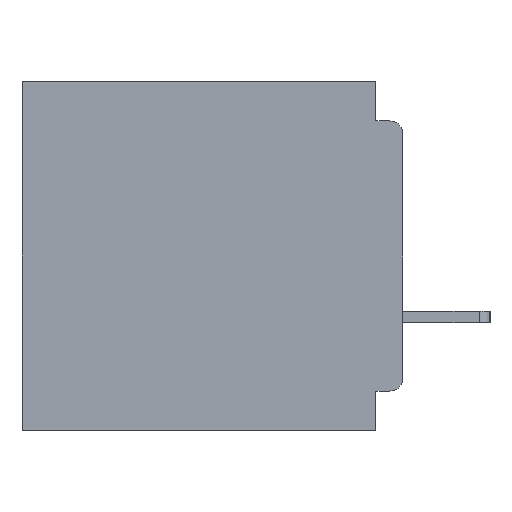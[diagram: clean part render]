
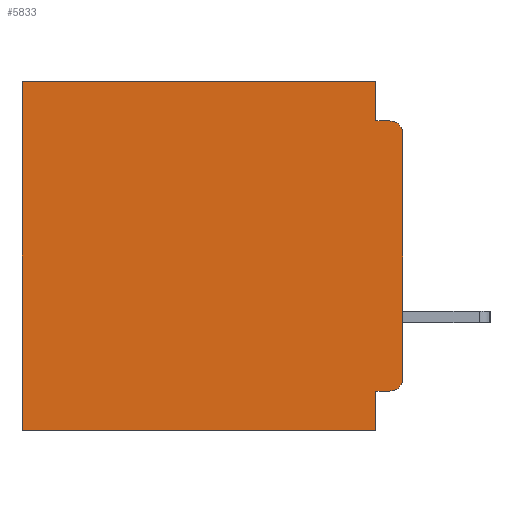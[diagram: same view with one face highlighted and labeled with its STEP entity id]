
A CAD part, left-side view. The second image highlights one B-rep face of the part: STEP entity #5833.
In plain terms, the highlighted planar face has unit normal (-1, 0, 0).
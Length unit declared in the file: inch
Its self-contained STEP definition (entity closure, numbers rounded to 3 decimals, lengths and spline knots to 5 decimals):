
#286 = VECTOR ( 'NONE', #21700, 39.37008 ) ;
#293 = LINE ( 'NONE', #2781, #18855 ) ;
#380 = LINE ( 'NONE', #12077, #38728 ) ;
#1965 = VERTEX_POINT ( 'NONE', #2530 ) ;
#2530 = CARTESIAN_POINT ( 'NONE',  ( 0.3, 0.031, -0.045 ) ) ;
#2781 = CARTESIAN_POINT ( 'NONE',  ( 0.3, 0., -0.045 ) ) ;
#3521 = ORIENTED_EDGE ( 'NONE', *, *, #38801, .F. ) ;
#3980 = DIRECTION ( 'NONE',  ( 0., 1., 0. ) ) ;
#4044 = VERTEX_POINT ( 'NONE', #16877 ) ;
#4296 = CARTESIAN_POINT ( 'NONE',  ( 0.3, 0.031, -0.4 ) ) ;
#4818 = LINE ( 'NONE', #4296, #43178 ) ;
#5797 = ORIENTED_EDGE ( 'NONE', *, *, #15759, .T. ) ;
#5833 = ADVANCED_FACE ( 'NONE', ( #33162 ), #35427, .F. ) ;
#5920 = CARTESIAN_POINT ( 'NONE',  ( 0.3, 0.437, 0. ) ) ;
#6751 = LINE ( 'NONE', #20584, #45153 ) ;
#6796 = CARTESIAN_POINT ( 'NONE',  ( 0.3, 0., -0.34 ) ) ;
#7523 = ORIENTED_EDGE ( 'NONE', *, *, #41508, .F. ) ;
#8393 = VERTEX_POINT ( 'NONE', #25454 ) ;
#8991 = VERTEX_POINT ( 'NONE', #25396 ) ;
#9329 = DIRECTION ( 'NONE',  ( 0., 0., -1. ) ) ;
#9753 = EDGE_CURVE ( 'NONE', #8991, #17204, #38625, .T. ) ;
#9806 = DIRECTION ( 'NONE',  ( -1., 0., 0. ) ) ;
#11230 = ORIENTED_EDGE ( 'NONE', *, *, #41575, .T. ) ;
#12008 = DIRECTION ( 'NONE',  ( 0., 1., 0. ) ) ;
#12077 = CARTESIAN_POINT ( 'NONE',  ( 0.3, 0., -0.4 ) ) ;
#13045 = VERTEX_POINT ( 'NONE', #5920 ) ;
#13140 = CARTESIAN_POINT ( 'NONE',  ( 0.3, 0., -0.4 ) ) ;
#13753 = VECTOR ( 'NONE', #43811, 39.37008 ) ;
#13840 = VERTEX_POINT ( 'NONE', #6796 ) ;
#15179 = EDGE_CURVE ( 'NONE', #13045, #17204, #16093, .T. ) ;
#15759 = EDGE_CURVE ( 'NONE', #23853, #8393, #46265, .T. ) ;
#16093 = LINE ( 'NONE', #40071, #13753 ) ;
#16729 = AXIS2_PLACEMENT_3D ( 'NONE', #18073, #44090, #21862 ) ;
#16877 = CARTESIAN_POINT ( 'NONE',  ( 0.3, 0.031, -0.355 ) ) ;
#16889 = DIRECTION ( 'NONE',  ( 1., 0., 0. ) ) ;
#17204 = VERTEX_POINT ( 'NONE', #30144 ) ;
#17555 = ORIENTED_EDGE ( 'NONE', *, *, #25535, .T. ) ;
#17685 = ORIENTED_EDGE ( 'NONE', *, *, #15179, .T. ) ;
#18073 = CARTESIAN_POINT ( 'NONE',  ( 0.3, 0.015, -0.06 ) ) ;
#18563 = VERTEX_POINT ( 'NONE', #29695 ) ;
#18712 = CARTESIAN_POINT ( 'NONE',  ( 0.3, 0., 0. ) ) ;
#18855 = VECTOR ( 'NONE', #25034, 39.37008 ) ;
#19042 = LINE ( 'NONE', #18712, #47535 ) ;
#20584 = CARTESIAN_POINT ( 'NONE',  ( 0.3, 0.031, 0. ) ) ;
#21700 = DIRECTION ( 'NONE',  ( 0., 1., 0. ) ) ;
#21789 = AXIS2_PLACEMENT_3D ( 'NONE', #32092, #9806, #35807 ) ;
#21862 = DIRECTION ( 'NONE',  ( 0., 0., -1. ) ) ;
#21966 = ORIENTED_EDGE ( 'NONE', *, *, #29088, .F. ) ;
#22521 = ORIENTED_EDGE ( 'NONE', *, *, #9753, .F. ) ;
#23246 = CARTESIAN_POINT ( 'NONE',  ( 0.3, 0., -0.355 ) ) ;
#23853 = VERTEX_POINT ( 'NONE', #23948 ) ;
#23948 = CARTESIAN_POINT ( 'NONE',  ( 0.3, 0., -0.06 ) ) ;
#25034 = DIRECTION ( 'NONE',  ( 0., -1., 0. ) ) ;
#25102 = EDGE_LOOP ( 'NONE', ( #3521, #5797, #29071, #7523, #17555, #17685, #22521, #21966, #26342, #11230 ) ) ;
#25396 = CARTESIAN_POINT ( 'NONE',  ( 0.3, 0.031, -0.4 ) ) ;
#25454 = CARTESIAN_POINT ( 'NONE',  ( 0.3, 0.015, -0.045 ) ) ;
#25535 = EDGE_CURVE ( 'NONE', #45112, #13045, #19042, .T. ) ;
#26342 = ORIENTED_EDGE ( 'NONE', *, *, #33182, .F. ) ;
#29071 = ORIENTED_EDGE ( 'NONE', *, *, #39721, .F. ) ;
#29088 = EDGE_CURVE ( 'NONE', #4044, #8991, #4818, .T. ) ;
#29156 = LINE ( 'NONE', #23246, #30287 ) ;
#29695 = CARTESIAN_POINT ( 'NONE',  ( 0.3, 0.015, -0.355 ) ) ;
#30144 = CARTESIAN_POINT ( 'NONE',  ( 0.3, 0.437, -0.4 ) ) ;
#30287 = VECTOR ( 'NONE', #12008, 39.37008 ) ;
#32092 = CARTESIAN_POINT ( 'NONE',  ( 0.3, 0.015, -0.34 ) ) ;
#32464 = AXIS2_PLACEMENT_3D ( 'NONE', #13140, #16889, #42892 ) ;
#33162 = FACE_OUTER_BOUND ( 'NONE', #25102, .T. ) ;
#33182 = EDGE_CURVE ( 'NONE', #18563, #4044, #29156, .T. ) ;
#35256 = CIRCLE ( 'NONE', #21789, 0.015 ) ;
#35427 = PLANE ( 'NONE',  #32464 ) ;
#35807 = DIRECTION ( 'NONE',  ( 0., 0., -1. ) ) ;
#37728 = DIRECTION ( 'NONE',  ( 0., 0., -1. ) ) ;
#38081 = DIRECTION ( 'NONE',  ( 0., 0., -1. ) ) ;
#38625 = LINE ( 'NONE', #43918, #286 ) ;
#38728 = VECTOR ( 'NONE', #38081, 39.37008 ) ;
#38801 = EDGE_CURVE ( 'NONE', #23853, #13840, #380, .T. ) ;
#39721 = EDGE_CURVE ( 'NONE', #1965, #8393, #293, .T. ) ;
#40071 = CARTESIAN_POINT ( 'NONE',  ( 0.3, 0.437, -0.4 ) ) ;
#40891 = CARTESIAN_POINT ( 'NONE',  ( 0.3, 0.031, 0. ) ) ;
#41508 = EDGE_CURVE ( 'NONE', #45112, #1965, #6751, .T. ) ;
#41575 = EDGE_CURVE ( 'NONE', #18563, #13840, #35256, .T. ) ;
#42892 = DIRECTION ( 'NONE',  ( 0., 0., -1. ) ) ;
#43178 = VECTOR ( 'NONE', #37728, 39.37008 ) ;
#43811 = DIRECTION ( 'NONE',  ( 0., 0., -1. ) ) ;
#43918 = CARTESIAN_POINT ( 'NONE',  ( 0.3, 0., -0.4 ) ) ;
#44090 = DIRECTION ( 'NONE',  ( -1., 0., 0. ) ) ;
#45112 = VERTEX_POINT ( 'NONE', #40891 ) ;
#45153 = VECTOR ( 'NONE', #9329, 39.37008 ) ;
#46265 = CIRCLE ( 'NONE', #16729, 0.015 ) ;
#47535 = VECTOR ( 'NONE', #3980, 39.37008 ) ;
